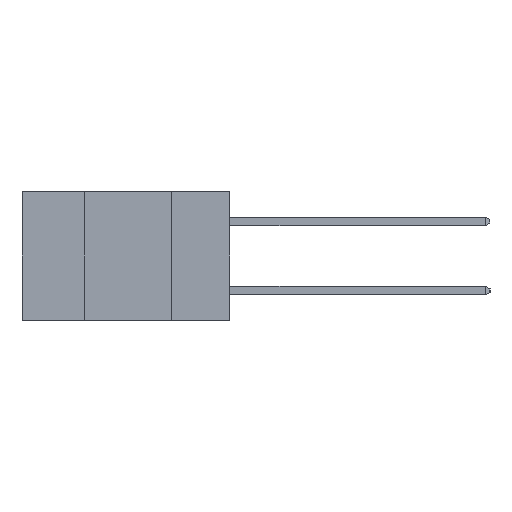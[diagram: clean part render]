
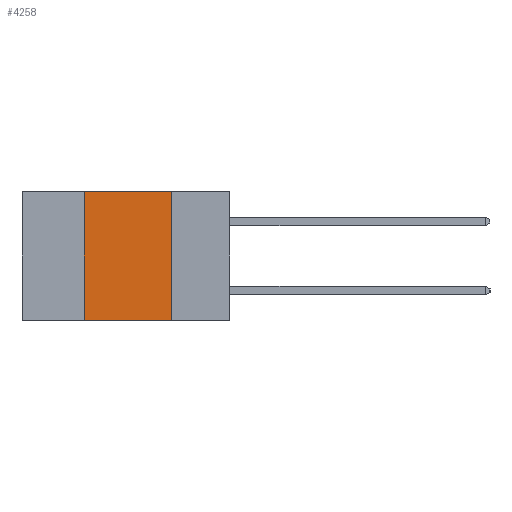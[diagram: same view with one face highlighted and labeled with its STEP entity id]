
A CAD part, left-side view. The second image highlights one B-rep face of the part: STEP entity #4258.
In plain terms, the highlighted planar face has unit normal (-1, 0, 0).
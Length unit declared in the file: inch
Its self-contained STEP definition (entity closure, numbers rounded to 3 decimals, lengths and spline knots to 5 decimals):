
#105 = EDGE_CURVE ( 'NONE', #1396, #4536, #6943, .T. ) ;
#514 = ORIENTED_EDGE ( 'NONE', *, *, #9748, .T. ) ;
#652 = VECTOR ( 'NONE', #16538, 39.37008 ) ;
#1074 = LINE ( 'NONE', #8945, #652 ) ;
#1396 = VERTEX_POINT ( 'NONE', #13746 ) ;
#2007 = EDGE_LOOP ( 'NONE', ( #3226, #7125, #10576, #514 ) ) ;
#2030 = LINE ( 'NONE', #7270, #14973 ) ;
#2245 = FACE_OUTER_BOUND ( 'NONE', #2007, .T. ) ;
#3226 = ORIENTED_EDGE ( 'NONE', *, *, #8822, .F. ) ;
#4258 = ADVANCED_FACE ( 'NONE', ( #2245 ), #12743, .F. ) ;
#4536 = VERTEX_POINT ( 'NONE', #8507 ) ;
#5463 = VERTEX_POINT ( 'NONE', #7614 ) ;
#6943 = LINE ( 'NONE', #16058, #16667 ) ;
#7125 = ORIENTED_EDGE ( 'NONE', *, *, #105, .F. ) ;
#7270 = CARTESIAN_POINT ( 'NONE',  ( 0., 0.6, -0.37 ) ) ;
#7487 = VERTEX_POINT ( 'NONE', #10412 ) ;
#7614 = CARTESIAN_POINT ( 'NONE',  ( 0., 0.17, -0.37 ) ) ;
#8507 = CARTESIAN_POINT ( 'NONE',  ( 0., 0.17, 0. ) ) ;
#8576 = DIRECTION ( 'NONE',  ( 0., 0., -1. ) ) ;
#8752 = DIRECTION ( 'NONE',  ( 0., -1., 0. ) ) ;
#8817 = AXIS2_PLACEMENT_3D ( 'NONE', #12736, #12402, #12350 ) ;
#8822 = EDGE_CURVE ( 'NONE', #4536, #5463, #12112, .T. ) ;
#8945 = CARTESIAN_POINT ( 'NONE',  ( 0., 0.42, -0.37 ) ) ;
#9161 = DIRECTION ( 'NONE',  ( 0., -1., 0. ) ) ;
#9478 = CARTESIAN_POINT ( 'NONE',  ( 0., 0.17, -0.37 ) ) ;
#9748 = EDGE_CURVE ( 'NONE', #7487, #5463, #2030, .T. ) ;
#10412 = CARTESIAN_POINT ( 'NONE',  ( 0., 0.42, -0.37 ) ) ;
#10576 = ORIENTED_EDGE ( 'NONE', *, *, #13335, .F. ) ;
#12112 = LINE ( 'NONE', #9478, #15402 ) ;
#12350 = DIRECTION ( 'NONE',  ( 0., 0., -1. ) ) ;
#12402 = DIRECTION ( 'NONE',  ( 1., 0., 0. ) ) ;
#12736 = CARTESIAN_POINT ( 'NONE',  ( 0., 0.6, 0. ) ) ;
#12743 = PLANE ( 'NONE',  #8817 ) ;
#13335 = EDGE_CURVE ( 'NONE', #7487, #1396, #1074, .T. ) ;
#13746 = CARTESIAN_POINT ( 'NONE',  ( 0., 0.42, 0. ) ) ;
#14973 = VECTOR ( 'NONE', #9161, 39.37008 ) ;
#15402 = VECTOR ( 'NONE', #8576, 39.37008 ) ;
#16058 = CARTESIAN_POINT ( 'NONE',  ( 0., 0.6, 0. ) ) ;
#16538 = DIRECTION ( 'NONE',  ( 0., 0., 1. ) ) ;
#16667 = VECTOR ( 'NONE', #8752, 39.37008 ) ;
